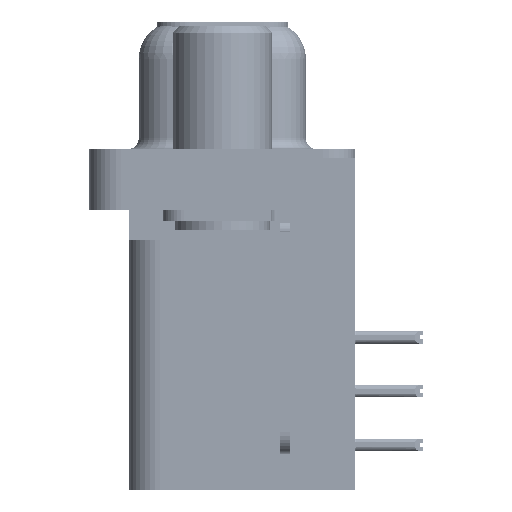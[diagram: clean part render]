
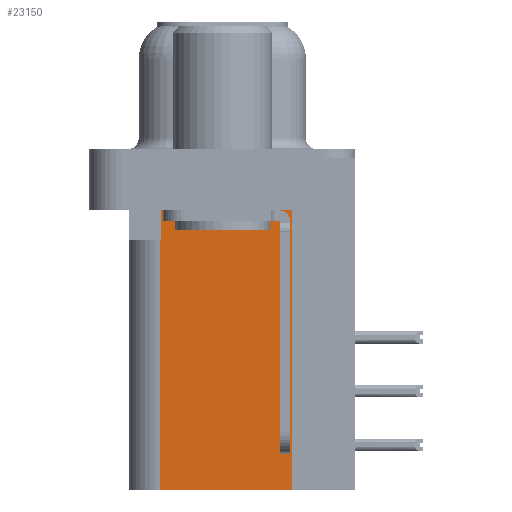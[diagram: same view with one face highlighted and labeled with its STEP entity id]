
A CAD part, left-side view. The second image highlights one B-rep face of the part: STEP entity #23150.
In plain terms, the highlighted planar face has unit normal (-1, 0, 0).
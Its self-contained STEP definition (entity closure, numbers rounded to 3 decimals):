
#125 = ORIENTED_EDGE ( 'NONE', *, *, #17008, .T. ) ;
#193 = EDGE_LOOP ( 'NONE', ( #28698, #34726, #6920, #16232, #4527, #125 ) ) ;
#2476 = VERTEX_POINT ( 'NONE', #46862 ) ;
#3803 = LINE ( 'NONE', #9913, #46046 ) ;
#4527 = ORIENTED_EDGE ( 'NONE', *, *, #47963, .F. ) ;
#4643 = DIRECTION ( 'NONE',  ( 0., 0., 1. ) ) ;
#4692 = AXIS2_PLACEMENT_3D ( 'NONE', #21298, #17342, #45992 ) ;
#4931 = EDGE_CURVE ( 'NONE', #49848, #13237, #22422, .T. ) ;
#5259 = VERTEX_POINT ( 'NONE', #27728 ) ;
#6920 = ORIENTED_EDGE ( 'NONE', *, *, #8083, .T. ) ;
#6979 = CARTESIAN_POINT ( 'NONE',  ( 3.79, 2.895, -2.5 ) ) ;
#7168 = LINE ( 'NONE', #41662, #50681 ) ;
#7482 = LINE ( 'NONE', #24981, #30468 ) ;
#8083 = EDGE_CURVE ( 'NONE', #19754, #32314, #14532, .T. ) ;
#9878 = VECTOR ( 'NONE', #12645, 1000. ) ;
#9913 = CARTESIAN_POINT ( 'NONE',  ( 3.79, 2.925, -15.7 ) ) ;
#10079 = DIRECTION ( 'NONE',  ( 0., 0., 1. ) ) ;
#11379 = CARTESIAN_POINT ( 'NONE',  ( 3.79, 2.925, -3.9 ) ) ;
#12645 = DIRECTION ( 'NONE',  ( 0., 0., -1. ) ) ;
#13075 = PLANE ( 'NONE',  #4692 ) ;
#13237 = VERTEX_POINT ( 'NONE', #6979 ) ;
#14532 = LINE ( 'NONE', #42562, #45896 ) ;
#14793 = CARTESIAN_POINT ( 'NONE',  ( 3.79, -3.295, -2.5 ) ) ;
#16232 = ORIENTED_EDGE ( 'NONE', *, *, #32729, .F. ) ;
#17008 = EDGE_CURVE ( 'NONE', #2476, #49848, #7482, .T. ) ;
#17103 = DIRECTION ( 'NONE',  ( 0., 1., 0. ) ) ;
#17342 = DIRECTION ( 'NONE',  ( 1., 0., 0. ) ) ;
#19754 = VERTEX_POINT ( 'NONE', #52925 ) ;
#20979 = CARTESIAN_POINT ( 'NONE',  ( 3.79, -3.295, -2.5 ) ) ;
#21298 = CARTESIAN_POINT ( 'NONE',  ( 3.79, -3.295, -15.7 ) ) ;
#22422 = LINE ( 'NONE', #20979, #45463 ) ;
#23150 = ADVANCED_FACE ( 'NONE', ( #24220 ), #13075, .F. ) ;
#24220 = FACE_OUTER_BOUND ( 'NONE', #193, .T. ) ;
#24981 = CARTESIAN_POINT ( 'NONE',  ( 3.79, -3.295, -15.7 ) ) ;
#27728 = CARTESIAN_POINT ( 'NONE',  ( 3.79, 2.925, -15.7 ) ) ;
#28698 = ORIENTED_EDGE ( 'NONE', *, *, #4931, .T. ) ;
#30308 = LINE ( 'NONE', #37189, #9878 ) ;
#30468 = VECTOR ( 'NONE', #4643, 1000. ) ;
#31872 = EDGE_CURVE ( 'NONE', #13237, #19754, #30308, .T. ) ;
#32314 = VERTEX_POINT ( 'NONE', #11379 ) ;
#32729 = EDGE_CURVE ( 'NONE', #5259, #32314, #3803, .T. ) ;
#34726 = ORIENTED_EDGE ( 'NONE', *, *, #31872, .T. ) ;
#37189 = CARTESIAN_POINT ( 'NONE',  ( 3.79, 2.895, -3.9 ) ) ;
#41406 = DIRECTION ( 'NONE',  ( 0., 1., 0. ) ) ;
#41662 = CARTESIAN_POINT ( 'NONE',  ( 3.79, -3.295, -15.7 ) ) ;
#42562 = CARTESIAN_POINT ( 'NONE',  ( 3.79, 0., -3.9 ) ) ;
#45463 = VECTOR ( 'NONE', #41406, 1000. ) ;
#45896 = VECTOR ( 'NONE', #46493, 1000. ) ;
#45992 = DIRECTION ( 'NONE',  ( 0., 0., -1. ) ) ;
#46046 = VECTOR ( 'NONE', #10079, 1000. ) ;
#46493 = DIRECTION ( 'NONE',  ( 0., 1., 0. ) ) ;
#46862 = CARTESIAN_POINT ( 'NONE',  ( 3.79, -3.295, -15.7 ) ) ;
#47963 = EDGE_CURVE ( 'NONE', #2476, #5259, #7168, .T. ) ;
#49848 = VERTEX_POINT ( 'NONE', #14793 ) ;
#50681 = VECTOR ( 'NONE', #17103, 1000. ) ;
#52925 = CARTESIAN_POINT ( 'NONE',  ( 3.79, 2.895, -3.9 ) ) ;
